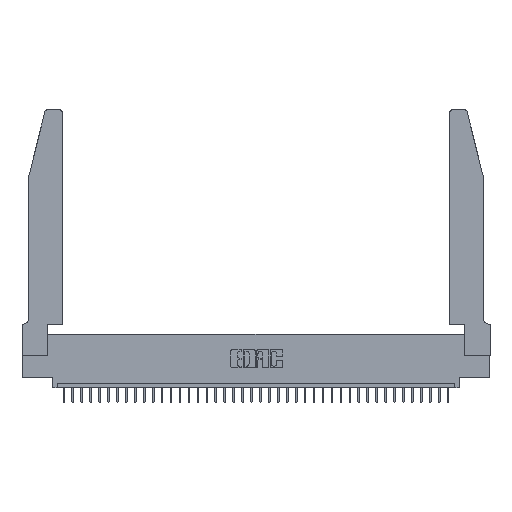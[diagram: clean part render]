
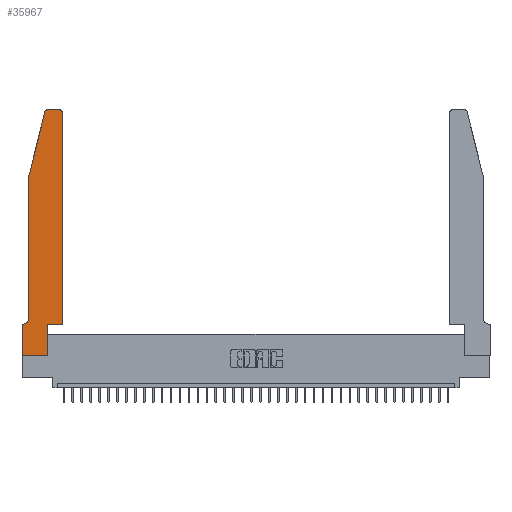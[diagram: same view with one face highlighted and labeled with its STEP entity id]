
A CAD part, top view. The second image highlights one B-rep face of the part: STEP entity #35967.
In plain terms, the highlighted planar face has unit normal (0, 0, 1).
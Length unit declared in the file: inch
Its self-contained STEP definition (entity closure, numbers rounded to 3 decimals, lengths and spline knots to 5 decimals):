
#338 = DIRECTION ( 'NONE',  ( -1., 0., 0. ) ) ;
#376 = CARTESIAN_POINT ( 'NONE',  ( 0.2865, 0.35, 0.37 ) ) ;
#402 = VERTEX_POINT ( 'NONE', #14498 ) ;
#860 = LINE ( 'NONE', #35781, #28804 ) ;
#1293 = VECTOR ( 'NONE', #24966, 39.37008 ) ;
#1992 = EDGE_CURVE ( 'NONE', #24979, #8482, #32872, .T. ) ;
#2370 = CARTESIAN_POINT ( 'NONE',  ( 0., 0., 0.37 ) ) ;
#2554 = AXIS2_PLACEMENT_3D ( 'NONE', #17896, #26582, #338 ) ;
#3174 = ORIENTED_EDGE ( 'NONE', *, *, #30980, .T. ) ;
#3771 = CARTESIAN_POINT ( 'NONE',  ( 0.284, 2.72, 0.37 ) ) ;
#4046 = EDGE_CURVE ( 'NONE', #8482, #18854, #34960, .T. ) ;
#4582 = CARTESIAN_POINT ( 'NONE',  ( 0.0755, 2., 0.37 ) ) ;
#4673 = LINE ( 'NONE', #4582, #16129 ) ;
#4908 = ORIENTED_EDGE ( 'NONE', *, *, #4046, .T. ) ;
#6142 = CARTESIAN_POINT ( 'NONE',  ( 0., 0., 0.37 ) ) ;
#6203 = CIRCLE ( 'NONE', #33143, 0.03 ) ;
#6410 = ORIENTED_EDGE ( 'NONE', *, *, #12696, .T. ) ;
#6948 = CARTESIAN_POINT ( 'NONE',  ( 0.4205, 2.72, 0.37 ) ) ;
#7439 = DIRECTION ( 'NONE',  ( 0., -1., 0. ) ) ;
#8482 = VERTEX_POINT ( 'NONE', #33517 ) ;
#8883 = FACE_OUTER_BOUND ( 'NONE', #16656, .T. ) ;
#9055 = EDGE_CURVE ( 'NONE', #18346, #402, #23886, .T. ) ;
#10245 = AXIS2_PLACEMENT_3D ( 'NONE', #6948, #21532, #27429 ) ;
#10413 = DIRECTION ( 'NONE',  ( 1., 0., 0. ) ) ;
#10892 = VERTEX_POINT ( 'NONE', #14638 ) ;
#10911 = ORIENTED_EDGE ( 'NONE', *, *, #24220, .T. ) ;
#10965 = CARTESIAN_POINT ( 'NONE',  ( 0.25487, 2.72718, 0.37 ) ) ;
#11317 = ORIENTED_EDGE ( 'NONE', *, *, #1992, .T. ) ;
#11323 = LINE ( 'NONE', #32643, #21805 ) ;
#12696 = EDGE_CURVE ( 'NONE', #26900, #17035, #11323, .T. ) ;
#12943 = LINE ( 'NONE', #2370, #18837 ) ;
#13252 = CARTESIAN_POINT ( 'NONE',  ( 0.2605, 2.75, 0.37 ) ) ;
#13384 = DIRECTION ( 'NONE',  ( -1., 0., 0. ) ) ;
#13564 = ORIENTED_EDGE ( 'NONE', *, *, #9055, .T. ) ;
#13577 = VECTOR ( 'NONE', #10413, 39.37008 ) ;
#14498 = CARTESIAN_POINT ( 'NONE',  ( 0.0755, 2., 0.37 ) ) ;
#14638 = CARTESIAN_POINT ( 'NONE',  ( 0.2865, 0.35, 0.37 ) ) ;
#14826 = AXIS2_PLACEMENT_3D ( 'NONE', #18008, #26950, #27085 ) ;
#15406 = ORIENTED_EDGE ( 'NONE', *, *, #23919, .T. ) ;
#16129 = VECTOR ( 'NONE', #18760, 39.37008 ) ;
#16529 = CARTESIAN_POINT ( 'NONE',  ( 0.4505, 0.35, 0.37 ) ) ;
#16573 = EDGE_CURVE ( 'NONE', #10892, #36592, #860, .T. ) ;
#16656 = EDGE_LOOP ( 'NONE', ( #4908, #15406, #13564, #31497, #25287, #6410, #31146, #10911, #35709, #28943, #3174, #11317 ) ) ;
#17035 = VERTEX_POINT ( 'NONE', #19066 ) ;
#17896 = CARTESIAN_POINT ( 'NONE',  ( 0.0055, 0.42, 0.37 ) ) ;
#18008 = CARTESIAN_POINT ( 'NONE',  ( 0., 0.35, 0.37 ) ) ;
#18346 = VERTEX_POINT ( 'NONE', #10965 ) ;
#18423 = VECTOR ( 'NONE', #37442, 39.37008 ) ;
#18760 = DIRECTION ( 'NONE',  ( 0., -1., 0. ) ) ;
#18837 = VECTOR ( 'NONE', #7439, 39.37008 ) ;
#18854 = VERTEX_POINT ( 'NONE', #20996 ) ;
#19066 = CARTESIAN_POINT ( 'NONE',  ( 0., 0.35, 0.37 ) ) ;
#19156 = CARTESIAN_POINT ( 'NONE',  ( 0.0755, 0.42, 0.37 ) ) ;
#19945 = VERTEX_POINT ( 'NONE', #19156 ) ;
#20122 = VERTEX_POINT ( 'NONE', #21743 ) ;
#20866 = EDGE_CURVE ( 'NONE', #402, #19945, #4673, .T. ) ;
#20996 = CARTESIAN_POINT ( 'NONE',  ( 0.284, 2.75, 0.37 ) ) ;
#21108 = EDGE_CURVE ( 'NONE', #17035, #24580, #12943, .T. ) ;
#21200 = PLANE ( 'NONE',  #14826 ) ;
#21403 = DIRECTION ( 'NONE',  ( 0., 0., 1. ) ) ;
#21442 = DIRECTION ( 'NONE',  ( -1., 0., 0. ) ) ;
#21532 = DIRECTION ( 'NONE',  ( 0., 0., 1. ) ) ;
#21743 = CARTESIAN_POINT ( 'NONE',  ( 0.2865, 0., 0.37 ) ) ;
#21805 = VECTOR ( 'NONE', #21442, 39.37008 ) ;
#23438 = EDGE_CURVE ( 'NONE', #20122, #10892, #33687, .T. ) ;
#23886 = LINE ( 'NONE', #29180, #18423 ) ;
#23919 = EDGE_CURVE ( 'NONE', #18854, #18346, #6203, .T. ) ;
#24220 = EDGE_CURVE ( 'NONE', #24580, #20122, #26343, .T. ) ;
#24580 = VERTEX_POINT ( 'NONE', #6142 ) ;
#24966 = DIRECTION ( 'NONE',  ( 0., 1., 0. ) ) ;
#24979 = VERTEX_POINT ( 'NONE', #27534 ) ;
#25230 = DIRECTION ( 'NONE',  ( 0., 1., 0. ) ) ;
#25287 = ORIENTED_EDGE ( 'NONE', *, *, #35906, .T. ) ;
#26343 = LINE ( 'NONE', #27531, #13577 ) ;
#26582 = DIRECTION ( 'NONE',  ( 0., 0., -1. ) ) ;
#26900 = VERTEX_POINT ( 'NONE', #36822 ) ;
#26950 = DIRECTION ( 'NONE',  ( 0., 0., 1. ) ) ;
#27085 = DIRECTION ( 'NONE',  ( 1., 0., 0. ) ) ;
#27429 = DIRECTION ( 'NONE',  ( 1., 0., 0. ) ) ;
#27520 = CARTESIAN_POINT ( 'NONE',  ( 0.4505, 0.35, 0.37 ) ) ;
#27531 = CARTESIAN_POINT ( 'NONE',  ( 0., 0., 0.37 ) ) ;
#27534 = CARTESIAN_POINT ( 'NONE',  ( 0.4505, 2.72, 0.37 ) ) ;
#27762 = DIRECTION ( 'NONE',  ( 1., 0., 0. ) ) ;
#28804 = VECTOR ( 'NONE', #27762, 39.37008 ) ;
#28943 = ORIENTED_EDGE ( 'NONE', *, *, #16573, .T. ) ;
#29180 = CARTESIAN_POINT ( 'NONE',  ( 0.0755, 2., 0.37 ) ) ;
#30980 = EDGE_CURVE ( 'NONE', #36592, #24979, #34629, .T. ) ;
#31146 = ORIENTED_EDGE ( 'NONE', *, *, #21108, .T. ) ;
#31497 = ORIENTED_EDGE ( 'NONE', *, *, #20866, .T. ) ;
#31780 = CIRCLE ( 'NONE', #2554, 0.07 ) ;
#32643 = CARTESIAN_POINT ( 'NONE',  ( 0.0755, 0.35, 0.37 ) ) ;
#32872 = CIRCLE ( 'NONE', #10245, 0.03 ) ;
#33143 = AXIS2_PLACEMENT_3D ( 'NONE', #3771, #21403, #35519 ) ;
#33517 = CARTESIAN_POINT ( 'NONE',  ( 0.4205, 2.75, 0.37 ) ) ;
#33687 = LINE ( 'NONE', #376, #36882 ) ;
#34526 = VECTOR ( 'NONE', #13384, 39.37008 ) ;
#34629 = LINE ( 'NONE', #16529, #1293 ) ;
#34960 = LINE ( 'NONE', #13252, #34526 ) ;
#35519 = DIRECTION ( 'NONE',  ( 1., 0., 0. ) ) ;
#35709 = ORIENTED_EDGE ( 'NONE', *, *, #23438, .T. ) ;
#35781 = CARTESIAN_POINT ( 'NONE',  ( 0.4505, 0.35, 0.37 ) ) ;
#35906 = EDGE_CURVE ( 'NONE', #19945, #26900, #31780, .T. ) ;
#35967 = ADVANCED_FACE ( 'NONE', ( #8883 ), #21200, .T. ) ;
#36592 = VERTEX_POINT ( 'NONE', #27520 ) ;
#36822 = CARTESIAN_POINT ( 'NONE',  ( 0.0055, 0.35, 0.37 ) ) ;
#36882 = VECTOR ( 'NONE', #25230, 39.37008 ) ;
#37442 = DIRECTION ( 'NONE',  ( -0.239, -0.971, 0. ) ) ;
